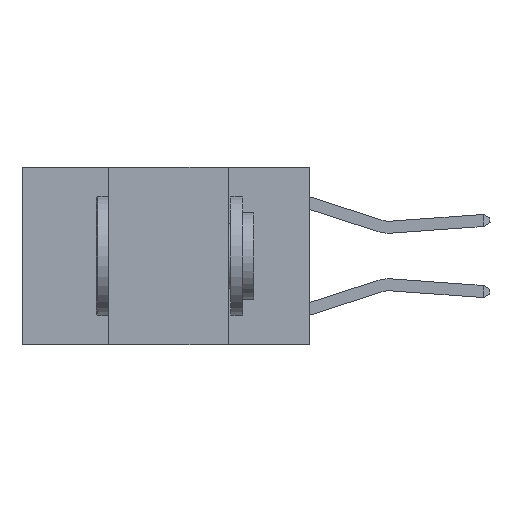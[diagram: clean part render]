
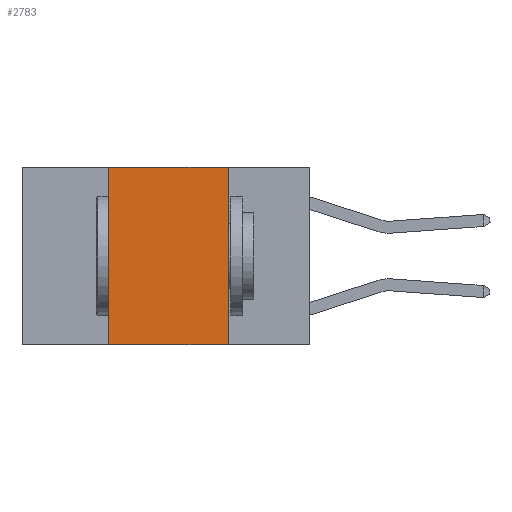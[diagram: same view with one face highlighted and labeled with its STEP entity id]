
A CAD part, left-side view. The second image highlights one B-rep face of the part: STEP entity #2783.
In plain terms, the highlighted planar face has unit normal (-1, 0, 0).
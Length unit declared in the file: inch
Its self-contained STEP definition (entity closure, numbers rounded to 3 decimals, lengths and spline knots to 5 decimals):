
#2266 = VERTEX_POINT ( 'NONE', #5563 ) ;
#2783 = ADVANCED_FACE ( 'NONE', ( #16234 ), #2959, .F. ) ;
#2959 = PLANE ( 'NONE',  #3001 ) ;
#3001 = AXIS2_PLACEMENT_3D ( 'NONE', #7399, #19362, #10343 ) ;
#3216 = EDGE_CURVE ( 'NONE', #8264, #2266, #5702, .T. ) ;
#3553 = LINE ( 'NONE', #7999, #14875 ) ;
#3830 = EDGE_LOOP ( 'NONE', ( #11224, #5940, #5611, #5110 ) ) ;
#4108 = VECTOR ( 'NONE', #7627, 39.37008 ) ;
#4469 = CARTESIAN_POINT ( 'NONE',  ( 0., 0.17, 0. ) ) ;
#5110 = ORIENTED_EDGE ( 'NONE', *, *, #3216, .T. ) ;
#5563 = CARTESIAN_POINT ( 'NONE',  ( 0., 0.17, -0.37 ) ) ;
#5611 = ORIENTED_EDGE ( 'NONE', *, *, #18492, .F. ) ;
#5702 = LINE ( 'NONE', #10415, #7726 ) ;
#5940 = ORIENTED_EDGE ( 'NONE', *, *, #14708, .F. ) ;
#6490 = EDGE_CURVE ( 'NONE', #17735, #2266, #3553, .T. ) ;
#6537 = DIRECTION ( 'NONE',  ( 0., 0., -1. ) ) ;
#6978 = DIRECTION ( 'NONE',  ( 0., 0., 1. ) ) ;
#7399 = CARTESIAN_POINT ( 'NONE',  ( 0., 0.6, 0. ) ) ;
#7627 = DIRECTION ( 'NONE',  ( 0., -1., 0. ) ) ;
#7726 = VECTOR ( 'NONE', #19339, 39.37008 ) ;
#7999 = CARTESIAN_POINT ( 'NONE',  ( 0., 0.17, 0. ) ) ;
#8264 = VERTEX_POINT ( 'NONE', #13139 ) ;
#10025 = LINE ( 'NONE', #14453, #15497 ) ;
#10343 = DIRECTION ( 'NONE',  ( 0., 0., -1. ) ) ;
#10415 = CARTESIAN_POINT ( 'NONE',  ( 0., 0.6, -0.37 ) ) ;
#11224 = ORIENTED_EDGE ( 'NONE', *, *, #6490, .F. ) ;
#11822 = CARTESIAN_POINT ( 'NONE',  ( 0., 0.42, 0. ) ) ;
#13139 = CARTESIAN_POINT ( 'NONE',  ( 0., 0.42, -0.37 ) ) ;
#14453 = CARTESIAN_POINT ( 'NONE',  ( 0., 0.42, 0. ) ) ;
#14708 = EDGE_CURVE ( 'NONE', #15205, #17735, #14877, .T. ) ;
#14875 = VECTOR ( 'NONE', #6537, 39.37008 ) ;
#14877 = LINE ( 'NONE', #18120, #4108 ) ;
#15205 = VERTEX_POINT ( 'NONE', #11822 ) ;
#15497 = VECTOR ( 'NONE', #6978, 39.37008 ) ;
#16234 = FACE_OUTER_BOUND ( 'NONE', #3830, .T. ) ;
#17735 = VERTEX_POINT ( 'NONE', #4469 ) ;
#18120 = CARTESIAN_POINT ( 'NONE',  ( 0., 0.6, 0. ) ) ;
#18492 = EDGE_CURVE ( 'NONE', #8264, #15205, #10025, .T. ) ;
#19339 = DIRECTION ( 'NONE',  ( 0., -1., 0. ) ) ;
#19362 = DIRECTION ( 'NONE',  ( 1., 0., 0. ) ) ;
